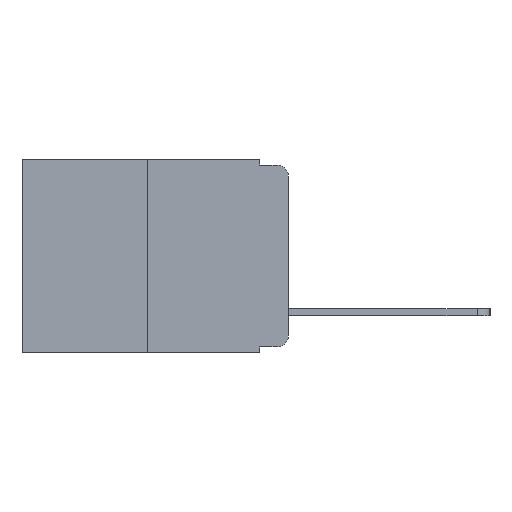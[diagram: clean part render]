
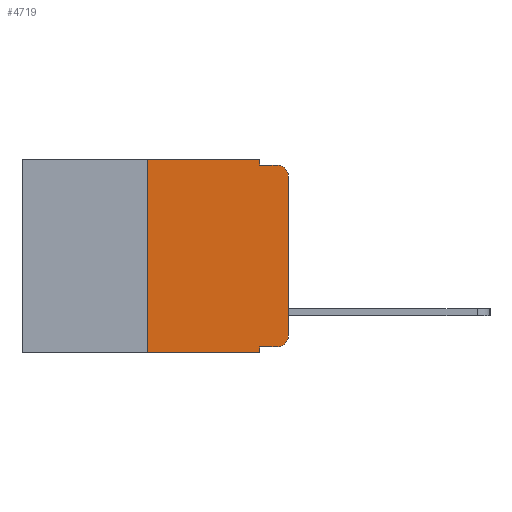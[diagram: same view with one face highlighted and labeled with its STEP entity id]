
A CAD part, left-side view. The second image highlights one B-rep face of the part: STEP entity #4719.
In plain terms, the highlighted planar face has unit normal (-1, 0, 0).
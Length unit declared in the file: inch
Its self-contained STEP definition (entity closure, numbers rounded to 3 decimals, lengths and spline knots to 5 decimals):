
#313 = ORIENTED_EDGE ( 'NONE', *, *, #16584, .T. ) ;
#409 = DIRECTION ( 'NONE',  ( 0., 0., -1. ) ) ;
#984 = CARTESIAN_POINT ( 'NONE',  ( 0., 0.051, -0.343 ) ) ;
#1344 = VERTEX_POINT ( 'NONE', #4168 ) ;
#1419 = CARTESIAN_POINT ( 'NONE',  ( 0., 0.02, -0.01 ) ) ;
#1446 = CIRCLE ( 'NONE', #18683, 0.02 ) ;
#1753 = CARTESIAN_POINT ( 'NONE',  ( 0., 0.02, -0.03 ) ) ;
#1947 = ORIENTED_EDGE ( 'NONE', *, *, #4074, .T. ) ;
#2237 = DIRECTION ( 'NONE',  ( 0., 0., -1. ) ) ;
#2288 = CARTESIAN_POINT ( 'NONE',  ( 0., 0.02, -0.333 ) ) ;
#2394 = VERTEX_POINT ( 'NONE', #2288 ) ;
#2395 = CARTESIAN_POINT ( 'NONE',  ( 0., 0.473, 0. ) ) ;
#2487 = VECTOR ( 'NONE', #12820, 39.37008 ) ;
#3186 = VERTEX_POINT ( 'NONE', #18141 ) ;
#3193 = EDGE_CURVE ( 'NONE', #13809, #9134, #8527, .T. ) ;
#3278 = CARTESIAN_POINT ( 'NONE',  ( 0., 0.473, -0.343 ) ) ;
#3338 = CARTESIAN_POINT ( 'NONE',  ( 0., 0.02, -0.313 ) ) ;
#3355 = LINE ( 'NONE', #7068, #14829 ) ;
#3458 = DIRECTION ( 'NONE',  ( 0., 0., -1. ) ) ;
#3656 = EDGE_CURVE ( 'NONE', #1344, #4022, #9163, .T. ) ;
#3850 = LINE ( 'NONE', #4015, #7496 ) ;
#4015 = CARTESIAN_POINT ( 'NONE',  ( 0., 0.051, -0.333 ) ) ;
#4022 = VERTEX_POINT ( 'NONE', #1419 ) ;
#4074 = EDGE_CURVE ( 'NONE', #3186, #9134, #18924, .T. ) ;
#4168 = CARTESIAN_POINT ( 'NONE',  ( 0., 0., -0.03 ) ) ;
#4719 = ADVANCED_FACE ( 'NONE', ( #4855 ), #6936, .F. ) ;
#4791 = ORIENTED_EDGE ( 'NONE', *, *, #3656, .T. ) ;
#4855 = FACE_OUTER_BOUND ( 'NONE', #7233, .T. ) ;
#4969 = DIRECTION ( 'NONE',  ( 0., 0., -1. ) ) ;
#5304 = ORIENTED_EDGE ( 'NONE', *, *, #18403, .F. ) ;
#6692 = EDGE_CURVE ( 'NONE', #3186, #12299, #11005, .T. ) ;
#6766 = ORIENTED_EDGE ( 'NONE', *, *, #3193, .F. ) ;
#6936 = PLANE ( 'NONE',  #15625 ) ;
#7011 = CARTESIAN_POINT ( 'NONE',  ( 0., 0., -0.313 ) ) ;
#7068 = CARTESIAN_POINT ( 'NONE',  ( 0., 0.051, 0. ) ) ;
#7216 = ORIENTED_EDGE ( 'NONE', *, *, #14626, .T. ) ;
#7233 = EDGE_LOOP ( 'NONE', ( #313, #4791, #8775, #5304, #13610, #17470, #1947, #6766, #7216, #14981 ) ) ;
#7439 = EDGE_CURVE ( 'NONE', #12299, #19440, #14721, .T. ) ;
#7496 = VECTOR ( 'NONE', #14439, 39.37008 ) ;
#8034 = DIRECTION ( 'NONE',  ( 0., 0., -1. ) ) ;
#8527 = LINE ( 'NONE', #19655, #15817 ) ;
#8775 = ORIENTED_EDGE ( 'NONE', *, *, #11741, .F. ) ;
#9134 = VERTEX_POINT ( 'NONE', #984 ) ;
#9163 = CIRCLE ( 'NONE', #12942, 0.02 ) ;
#9779 = CARTESIAN_POINT ( 'NONE',  ( 0., 0.25, 0. ) ) ;
#9807 = DIRECTION ( 'NONE',  ( 1., 0., 0. ) ) ;
#10129 = DIRECTION ( 'NONE',  ( 0., -1., 0. ) ) ;
#11005 = LINE ( 'NONE', #9779, #2487 ) ;
#11115 = CARTESIAN_POINT ( 'NONE',  ( 0., 0.051, -0.01 ) ) ;
#11428 = DIRECTION ( 'NONE',  ( 0., -1., 0. ) ) ;
#11563 = LINE ( 'NONE', #13733, #14903 ) ;
#11741 = EDGE_CURVE ( 'NONE', #19620, #4022, #18820, .T. ) ;
#12299 = VERTEX_POINT ( 'NONE', #13656 ) ;
#12424 = DIRECTION ( 'NONE',  ( -1., 0., 0. ) ) ;
#12653 = CARTESIAN_POINT ( 'NONE',  ( 0., 0.473, 0. ) ) ;
#12820 = DIRECTION ( 'NONE',  ( 0., 0., 1. ) ) ;
#12942 = AXIS2_PLACEMENT_3D ( 'NONE', #1753, #12424, #3458 ) ;
#13610 = ORIENTED_EDGE ( 'NONE', *, *, #7439, .F. ) ;
#13656 = CARTESIAN_POINT ( 'NONE',  ( 0., 0.25, 0. ) ) ;
#13733 = CARTESIAN_POINT ( 'NONE',  ( 0., 0., 0. ) ) ;
#13809 = VERTEX_POINT ( 'NONE', #18753 ) ;
#13835 = DIRECTION ( 'NONE',  ( -1., 0., 0. ) ) ;
#14439 = DIRECTION ( 'NONE',  ( 0., -1., 0. ) ) ;
#14499 = VECTOR ( 'NONE', #10129, 39.37008 ) ;
#14526 = CARTESIAN_POINT ( 'NONE',  ( 0., 0.051, -0.01 ) ) ;
#14626 = EDGE_CURVE ( 'NONE', #13809, #2394, #3850, .T. ) ;
#14721 = LINE ( 'NONE', #2395, #18128 ) ;
#14829 = VECTOR ( 'NONE', #2237, 39.37008 ) ;
#14903 = VECTOR ( 'NONE', #18103, 39.37008 ) ;
#14981 = ORIENTED_EDGE ( 'NONE', *, *, #15672, .T. ) ;
#15073 = VECTOR ( 'NONE', #15240, 39.37008 ) ;
#15220 = CARTESIAN_POINT ( 'NONE',  ( 0., 0.051, 0. ) ) ;
#15240 = DIRECTION ( 'NONE',  ( 0., -1., 0. ) ) ;
#15625 = AXIS2_PLACEMENT_3D ( 'NONE', #12653, #9807, #409 ) ;
#15672 = EDGE_CURVE ( 'NONE', #2394, #18357, #1446, .T. ) ;
#15817 = VECTOR ( 'NONE', #8034, 39.37008 ) ;
#16584 = EDGE_CURVE ( 'NONE', #18357, #1344, #11563, .T. ) ;
#17470 = ORIENTED_EDGE ( 'NONE', *, *, #6692, .F. ) ;
#18103 = DIRECTION ( 'NONE',  ( 0., 0., 1. ) ) ;
#18128 = VECTOR ( 'NONE', #11428, 39.37008 ) ;
#18141 = CARTESIAN_POINT ( 'NONE',  ( 0., 0.25, -0.343 ) ) ;
#18357 = VERTEX_POINT ( 'NONE', #7011 ) ;
#18403 = EDGE_CURVE ( 'NONE', #19440, #19620, #3355, .T. ) ;
#18683 = AXIS2_PLACEMENT_3D ( 'NONE', #3338, #13835, #4969 ) ;
#18753 = CARTESIAN_POINT ( 'NONE',  ( 0., 0.051, -0.333 ) ) ;
#18820 = LINE ( 'NONE', #14526, #14499 ) ;
#18924 = LINE ( 'NONE', #3278, #15073 ) ;
#19440 = VERTEX_POINT ( 'NONE', #15220 ) ;
#19620 = VERTEX_POINT ( 'NONE', #11115 ) ;
#19655 = CARTESIAN_POINT ( 'NONE',  ( 0., 0.051, 0. ) ) ;
